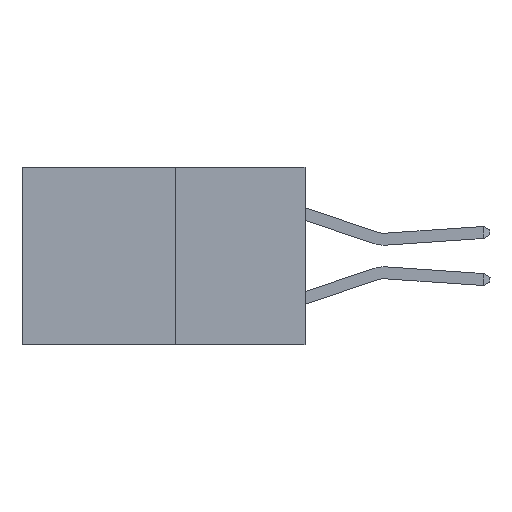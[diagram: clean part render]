
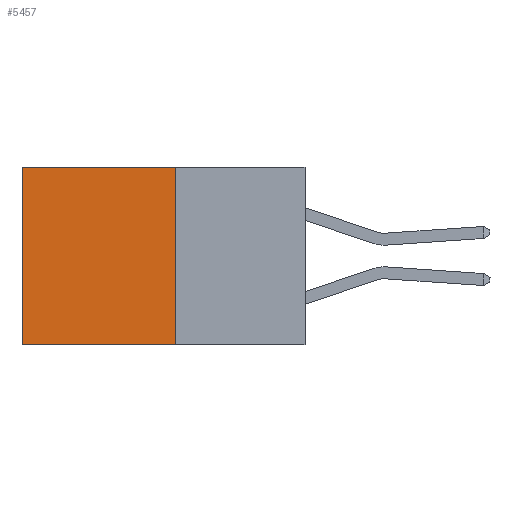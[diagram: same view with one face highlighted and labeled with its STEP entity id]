
A CAD part, left-side view. The second image highlights one B-rep face of the part: STEP entity #5457.
In plain terms, the highlighted planar face has unit normal (-1, 0, 0).
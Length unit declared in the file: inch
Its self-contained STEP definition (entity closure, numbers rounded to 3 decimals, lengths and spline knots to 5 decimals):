
#71 = ORIENTED_EDGE ( 'NONE', *, *, #9511, .F. ) ;
#79 = ORIENTED_EDGE ( 'NONE', *, *, #5516, .F. ) ;
#339 = ORIENTED_EDGE ( 'NONE', *, *, #3024, .T. ) ;
#1320 = VECTOR ( 'NONE', #3031, 39.37008 ) ;
#1876 = VERTEX_POINT ( 'NONE', #7799 ) ;
#2288 = VERTEX_POINT ( 'NONE', #11852 ) ;
#2685 = VECTOR ( 'NONE', #3167, 39.37008 ) ;
#2974 = LINE ( 'NONE', #3437, #2685 ) ;
#3012 = VERTEX_POINT ( 'NONE', #7985 ) ;
#3024 = EDGE_CURVE ( 'NONE', #1876, #3012, #6800, .T. ) ;
#3031 = DIRECTION ( 'NONE',  ( 0., 1., 0. ) ) ;
#3167 = DIRECTION ( 'NONE',  ( 0., 1., 0. ) ) ;
#3437 = CARTESIAN_POINT ( 'NONE',  ( 0.277, 0.27, -0.37 ) ) ;
#3905 = VECTOR ( 'NONE', #8236, 39.37008 ) ;
#4083 = LINE ( 'NONE', #9027, #9220 ) ;
#4142 = EDGE_LOOP ( 'NONE', ( #4429, #71, #79, #339 ) ) ;
#4429 = ORIENTED_EDGE ( 'NONE', *, *, #9012, .T. ) ;
#5282 = VERTEX_POINT ( 'NONE', #11290 ) ;
#5457 = ADVANCED_FACE ( 'NONE', ( #7934 ), #9739, .F. ) ;
#5516 = EDGE_CURVE ( 'NONE', #1876, #5282, #4083, .T. ) ;
#5913 = AXIS2_PLACEMENT_3D ( 'NONE', #9750, #9663, #9647 ) ;
#6613 = CARTESIAN_POINT ( 'NONE',  ( 0.277, 0.27, 0. ) ) ;
#6800 = LINE ( 'NONE', #6613, #1320 ) ;
#7799 = CARTESIAN_POINT ( 'NONE',  ( 0.277, 0.27, 0. ) ) ;
#7934 = FACE_OUTER_BOUND ( 'NONE', #4142, .T. ) ;
#7985 = CARTESIAN_POINT ( 'NONE',  ( 0.277, 0.59, 0. ) ) ;
#8193 = CARTESIAN_POINT ( 'NONE',  ( 0.277, 0.59, -0.37 ) ) ;
#8236 = DIRECTION ( 'NONE',  ( 0., 0., -1. ) ) ;
#9012 = EDGE_CURVE ( 'NONE', #3012, #2288, #9051, .T. ) ;
#9027 = CARTESIAN_POINT ( 'NONE',  ( 0.277, 0.27, -0.37 ) ) ;
#9051 = LINE ( 'NONE', #8193, #3905 ) ;
#9080 = DIRECTION ( 'NONE',  ( 0., 0., -1. ) ) ;
#9220 = VECTOR ( 'NONE', #9080, 39.37008 ) ;
#9511 = EDGE_CURVE ( 'NONE', #5282, #2288, #2974, .T. ) ;
#9647 = DIRECTION ( 'NONE',  ( 0., 0., -1. ) ) ;
#9663 = DIRECTION ( 'NONE',  ( 1., 0., 0. ) ) ;
#9739 = PLANE ( 'NONE',  #5913 ) ;
#9750 = CARTESIAN_POINT ( 'NONE',  ( 0.277, 0.27, -0.37 ) ) ;
#11290 = CARTESIAN_POINT ( 'NONE',  ( 0.277, 0.27, -0.37 ) ) ;
#11852 = CARTESIAN_POINT ( 'NONE',  ( 0.277, 0.59, -0.37 ) ) ;
